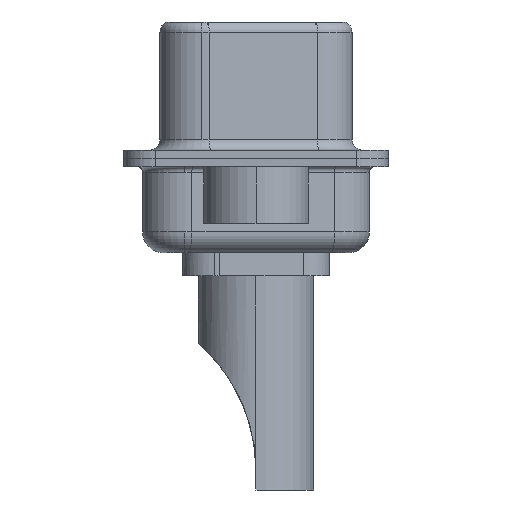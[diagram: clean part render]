
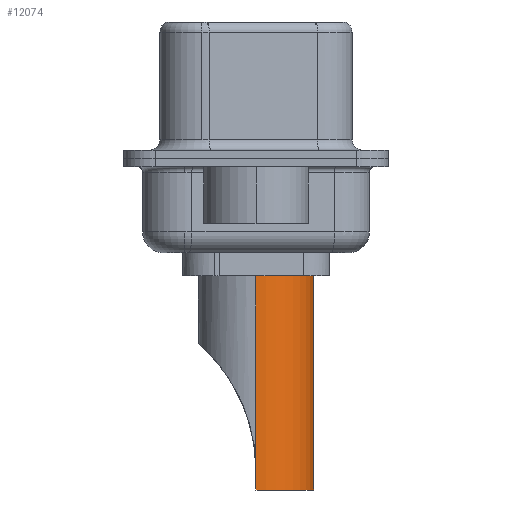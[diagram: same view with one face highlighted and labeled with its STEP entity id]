
A CAD part, left-side view. The second image highlights one B-rep face of the part: STEP entity #12074.
In plain terms, the highlighted cylindrical face has radius 2.75 mm (diameter 5.5 mm), a partial arc.
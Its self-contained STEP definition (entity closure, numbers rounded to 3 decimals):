
#459 = EDGE_CURVE ( 'NONE', #18387, #13570, #5864, .T. ) ;
#604 = ORIENTED_EDGE ( 'NONE', *, *, #459, .F. ) ;
#816 = CARTESIAN_POINT ( 'NONE',  ( -2.75, 0., -7.764 ) ) ;
#884 = CARTESIAN_POINT ( 'NONE',  ( 0., 0., 1.5 ) ) ;
#1653 = EDGE_CURVE ( 'NONE', #13570, #7737, #17874, .T. ) ;
#1797 = CARTESIAN_POINT ( 'NONE',  ( 2.75, 0., -8.7 ) ) ;
#3711 = LINE ( 'NONE', #6569, #8291 ) ;
#4022 = DIRECTION ( 'NONE',  ( 0., 0., -1. ) ) ;
#4041 = EDGE_LOOP ( 'NONE', ( #604, #12821, #19300, #7129, #4623, #16897 ) ) ;
#4123 = EDGE_CURVE ( 'NONE', #13472, #9337, #15921, .T. ) ;
#4463 = LINE ( 'NONE', #8761, #8986 ) ;
#4623 = ORIENTED_EDGE ( 'NONE', *, *, #18724, .T. ) ;
#5080 = FACE_OUTER_BOUND ( 'NONE', #4041, .T. ) ;
#5864 = LINE ( 'NONE', #18168, #18971 ) ;
#6569 = CARTESIAN_POINT ( 'NONE',  ( 2.75, 0., -8.7 ) ) ;
#7129 = ORIENTED_EDGE ( 'NONE', *, *, #16305, .F. ) ;
#7737 = VERTEX_POINT ( 'NONE', #15245 ) ;
#7982 = DIRECTION ( 'NONE',  ( 0., 0., 1. ) ) ;
#8001 = EDGE_CURVE ( 'NONE', #18387, #13472, #12621, .T. ) ;
#8291 = VECTOR ( 'NONE', #13380, 1000. ) ;
#8642 = VECTOR ( 'NONE', #4022, 1000. ) ;
#8761 = CARTESIAN_POINT ( 'NONE',  ( 2.75, 0., 4.234 ) ) ;
#8986 = VECTOR ( 'NONE', #19028, 1000. ) ;
#9337 = VERTEX_POINT ( 'NONE', #1797 ) ;
#10384 = CARTESIAN_POINT ( 'NONE',  ( 0., 0., -8.7 ) ) ;
#11625 = DIRECTION ( 'NONE',  ( 0., 0., 1. ) ) ;
#11798 = AXIS2_PLACEMENT_3D ( 'NONE', #884, #18398, #18327 ) ;
#12074 = ADVANCED_FACE ( 'NONE', ( #5080 ), #13581, .T. ) ;
#12621 = LINE ( 'NONE', #14262, #8642 ) ;
#12821 = ORIENTED_EDGE ( 'NONE', *, *, #8001, .T. ) ;
#12844 = CARTESIAN_POINT ( 'NONE',  ( -2.75, 0., 1.5 ) ) ;
#13380 = DIRECTION ( 'NONE',  ( 0., 0., -1. ) ) ;
#13472 = VERTEX_POINT ( 'NONE', #13981 ) ;
#13570 = VERTEX_POINT ( 'NONE', #12844 ) ;
#13581 = CYLINDRICAL_SURFACE ( 'NONE', #21865, 2.75 ) ;
#13981 = CARTESIAN_POINT ( 'NONE',  ( -2.75, 0., -8.7 ) ) ;
#14262 = CARTESIAN_POINT ( 'NONE',  ( -2.75, 0., -8.7 ) ) ;
#15245 = CARTESIAN_POINT ( 'NONE',  ( 2.75, 0., 1.5 ) ) ;
#15921 = CIRCLE ( 'NONE', #19915, 2.75 ) ;
#16305 = EDGE_CURVE ( 'NONE', #18566, #9337, #3711, .T. ) ;
#16422 = CARTESIAN_POINT ( 'NONE',  ( 0., 0., 4.234 ) ) ;
#16897 = ORIENTED_EDGE ( 'NONE', *, *, #1653, .F. ) ;
#17874 = CIRCLE ( 'NONE', #11798, 2.75 ) ;
#18168 = CARTESIAN_POINT ( 'NONE',  ( -2.75, 0., 4.234 ) ) ;
#18239 = DIRECTION ( 'NONE',  ( 1., 0., 0. ) ) ;
#18327 = DIRECTION ( 'NONE',  ( 1., 0., 0. ) ) ;
#18387 = VERTEX_POINT ( 'NONE', #816 ) ;
#18398 = DIRECTION ( 'NONE',  ( 0., 0., 1. ) ) ;
#18566 = VERTEX_POINT ( 'NONE', #21887 ) ;
#18724 = EDGE_CURVE ( 'NONE', #18566, #7737, #4463, .T. ) ;
#18971 = VECTOR ( 'NONE', #21373, 1000. ) ;
#19028 = DIRECTION ( 'NONE',  ( 0., 0., 1. ) ) ;
#19300 = ORIENTED_EDGE ( 'NONE', *, *, #4123, .T. ) ;
#19915 = AXIS2_PLACEMENT_3D ( 'NONE', #10384, #11625, #21236 ) ;
#21236 = DIRECTION ( 'NONE',  ( 1., 0., 0. ) ) ;
#21373 = DIRECTION ( 'NONE',  ( 0., 0., 1. ) ) ;
#21865 = AXIS2_PLACEMENT_3D ( 'NONE', #16422, #7982, #18239 ) ;
#21887 = CARTESIAN_POINT ( 'NONE',  ( 2.75, 0., -7.764 ) ) ;
